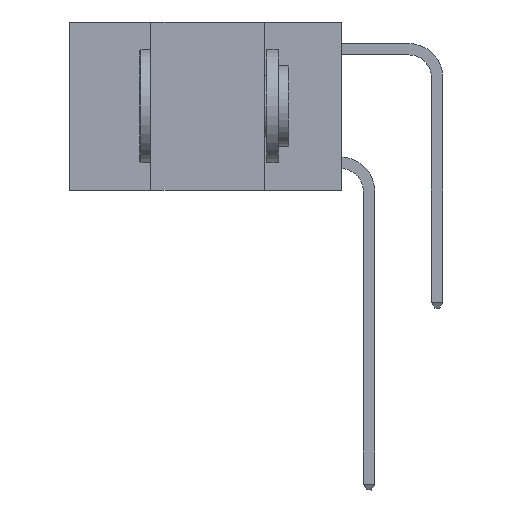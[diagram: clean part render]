
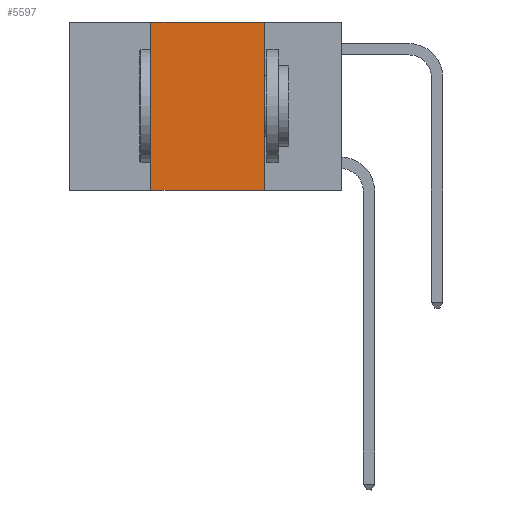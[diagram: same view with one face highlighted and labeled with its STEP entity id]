
A CAD part, left-side view. The second image highlights one B-rep face of the part: STEP entity #5597.
In plain terms, the highlighted planar face has unit normal (-1, 0, 0).
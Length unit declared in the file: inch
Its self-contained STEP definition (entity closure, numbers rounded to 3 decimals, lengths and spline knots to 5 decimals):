
#843 = CARTESIAN_POINT ( 'NONE',  ( 0., 0.6, 0. ) ) ;
#884 = CARTESIAN_POINT ( 'NONE',  ( 0., 0.42, 0. ) ) ;
#2033 = AXIS2_PLACEMENT_3D ( 'NONE', #843, #2774, #13177 ) ;
#2168 = LINE ( 'NONE', #2550, #6514 ) ;
#2224 = EDGE_LOOP ( 'NONE', ( #20934, #13732, #4692, #11942 ) ) ;
#2550 = CARTESIAN_POINT ( 'NONE',  ( 0., 0.17, 0. ) ) ;
#2584 = LINE ( 'NONE', #15756, #11207 ) ;
#2774 = DIRECTION ( 'NONE',  ( 1., 0., 0. ) ) ;
#3189 = CARTESIAN_POINT ( 'NONE',  ( 0., 0.17, 0. ) ) ;
#3414 = VERTEX_POINT ( 'NONE', #21370 ) ;
#4692 = ORIENTED_EDGE ( 'NONE', *, *, #8729, .F. ) ;
#5538 = LINE ( 'NONE', #14124, #21839 ) ;
#5562 = DIRECTION ( 'NONE',  ( 0., -1., 0. ) ) ;
#5597 = ADVANCED_FACE ( 'NONE', ( #15216 ), #11485, .F. ) ;
#6514 = VECTOR ( 'NONE', #21259, 39.37008 ) ;
#7075 = VECTOR ( 'NONE', #19426, 39.37008 ) ;
#7343 = EDGE_CURVE ( 'NONE', #3414, #17404, #2584, .T. ) ;
#7444 = CARTESIAN_POINT ( 'NONE',  ( 0., 0.6, 0. ) ) ;
#8729 = EDGE_CURVE ( 'NONE', #3414, #15039, #5538, .T. ) ;
#8939 = VERTEX_POINT ( 'NONE', #3189 ) ;
#9456 = EDGE_CURVE ( 'NONE', #15039, #8939, #14045, .T. ) ;
#11207 = VECTOR ( 'NONE', #5562, 39.37008 ) ;
#11485 = PLANE ( 'NONE',  #2033 ) ;
#11942 = ORIENTED_EDGE ( 'NONE', *, *, #7343, .T. ) ;
#12111 = DIRECTION ( 'NONE',  ( 0., 0., 1. ) ) ;
#13177 = DIRECTION ( 'NONE',  ( 0., 0., -1. ) ) ;
#13732 = ORIENTED_EDGE ( 'NONE', *, *, #9456, .F. ) ;
#14045 = LINE ( 'NONE', #7444, #7075 ) ;
#14124 = CARTESIAN_POINT ( 'NONE',  ( 0., 0.42, 0. ) ) ;
#15039 = VERTEX_POINT ( 'NONE', #884 ) ;
#15216 = FACE_OUTER_BOUND ( 'NONE', #2224, .T. ) ;
#15756 = CARTESIAN_POINT ( 'NONE',  ( 0., 0.6, -0.37 ) ) ;
#17404 = VERTEX_POINT ( 'NONE', #20485 ) ;
#19426 = DIRECTION ( 'NONE',  ( 0., -1., 0. ) ) ;
#20485 = CARTESIAN_POINT ( 'NONE',  ( 0., 0.17, -0.37 ) ) ;
#20874 = EDGE_CURVE ( 'NONE', #8939, #17404, #2168, .T. ) ;
#20934 = ORIENTED_EDGE ( 'NONE', *, *, #20874, .F. ) ;
#21259 = DIRECTION ( 'NONE',  ( 0., 0., -1. ) ) ;
#21370 = CARTESIAN_POINT ( 'NONE',  ( 0., 0.42, -0.37 ) ) ;
#21839 = VECTOR ( 'NONE', #12111, 39.37008 ) ;
